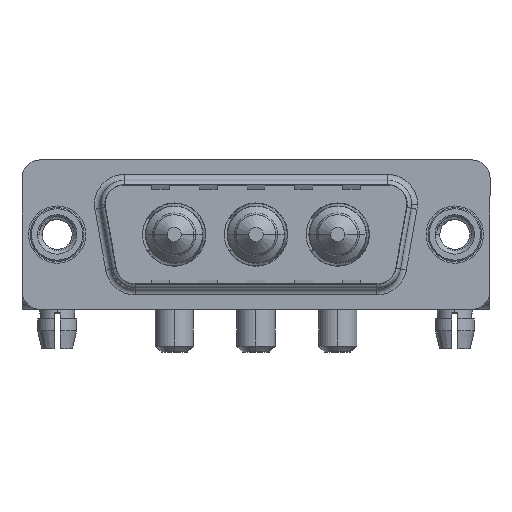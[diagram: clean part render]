
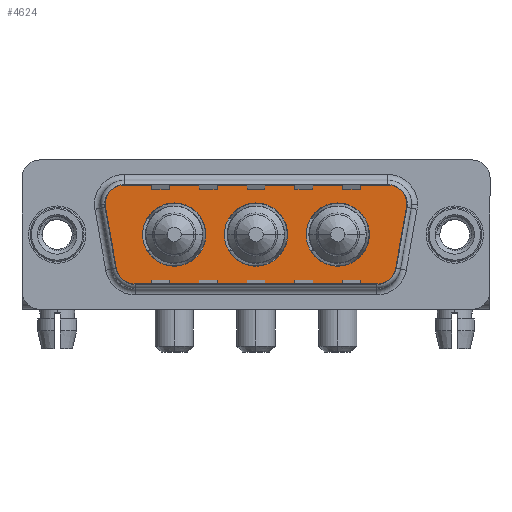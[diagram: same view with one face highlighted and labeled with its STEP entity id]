
A CAD part, top view. The second image highlights one B-rep face of the part: STEP entity #4624.
In plain terms, the highlighted planar face has unit normal (0, 0, 1).
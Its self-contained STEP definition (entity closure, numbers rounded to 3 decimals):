
#15 = EDGE_CURVE ( 'NONE', #15211, #13319, #9795, .T. ) ;
#98 = CARTESIAN_POINT ( 'NONE',  ( 5.411, 4.9, 0. ) ) ;
#566 = CIRCLE ( 'NONE', #9635, 2.65 ) ;
#804 = CARTESIAN_POINT ( 'NONE',  ( 4.464, -3.247, 0. ) ) ;
#961 = ORIENTED_EDGE ( 'NONE', *, *, #15995, .T. ) ;
#1162 = EDGE_LOOP ( 'NONE', ( #7619, #8279 ) ) ;
#1176 = ORIENTED_EDGE ( 'NONE', *, *, #10831, .T. ) ;
#1302 = DIRECTION ( 'NONE',  ( 0., 0., 1. ) ) ;
#1475 = EDGE_LOOP ( 'NONE', ( #9793, #8203 ) ) ;
#1520 = DIRECTION ( 'NONE',  ( 0., 0., 1. ) ) ;
#1812 = DIRECTION ( 'NONE',  ( 0., 0., 1. ) ) ;
#1900 = DIRECTION ( 'NONE',  ( 1., 0., 0. ) ) ;
#2204 = EDGE_CURVE ( 'NONE', #5105, #12135, #5934, .T. ) ;
#2297 = EDGE_CURVE ( 'NONE', #10391, #4183, #5661, .T. ) ;
#2346 = PLANE ( 'NONE',  #7996 ) ;
#2433 = EDGE_CURVE ( 'NONE', #5829, #15723, #12809, .T. ) ;
#2524 = CARTESIAN_POINT ( 'NONE',  ( 20.85, 0., 0. ) ) ;
#2596 = DIRECTION ( 'NONE',  ( 1., 0., 0. ) ) ;
#2720 = ORIENTED_EDGE ( 'NONE', *, *, #14276, .F. ) ;
#3393 = CARTESIAN_POINT ( 'NONE',  ( 23.5, 0., 0. ) ) ;
#3541 = VECTOR ( 'NONE', #15033, 1000. ) ;
#3607 = EDGE_CURVE ( 'NONE', #12135, #5105, #566, .T. ) ;
#3688 = DIRECTION ( 'NONE',  ( -1., 0., 0. ) ) ;
#3968 = FACE_BOUND ( 'NONE', #1475, .T. ) ;
#4048 = DIRECTION ( 'NONE',  ( 1., 0., 0. ) ) ;
#4058 = AXIS2_PLACEMENT_3D ( 'NONE', #6851, #8571, #6929 ) ;
#4127 = DIRECTION ( 'NONE',  ( 1., 0., 0. ) ) ;
#4183 = VERTEX_POINT ( 'NONE', #2524 ) ;
#4293 = CARTESIAN_POINT ( 'NONE',  ( 9.8, 0., 0. ) ) ;
#4350 = CARTESIAN_POINT ( 'NONE',  ( 9.8, 0., 0. ) ) ;
#4551 = VECTOR ( 'NONE', #9994, 1000. ) ;
#4624 = ADVANCED_FACE ( 'NONE', ( #3968, #9059, #15495, #14115 ), #2346, .T. ) ;
#4654 = DIRECTION ( 'NONE',  ( 1., 0., 0. ) ) ;
#4661 = AXIS2_PLACEMENT_3D ( 'NONE', #10235, #7649, #3688 ) ;
#4957 = ORIENTED_EDGE ( 'NONE', *, *, #14246, .T. ) ;
#5105 = VERTEX_POINT ( 'NONE', #8069 ) ;
#5158 = CARTESIAN_POINT ( 'NONE',  ( 6.434, -4.9, 0. ) ) ;
#5204 = CARTESIAN_POINT ( 'NONE',  ( 16.65, 0., 0. ) ) ;
#5661 = CIRCLE ( 'NONE', #10350, 2.65 ) ;
#5746 = EDGE_LOOP ( 'NONE', ( #15866, #4957, #961, #13502, #1176, #6097, #14659, #13693, #10417 ) ) ;
#5797 = DIRECTION ( 'NONE',  ( 1., 0., 0. ) ) ;
#5829 = VERTEX_POINT ( 'NONE', #9871 ) ;
#5934 = CIRCLE ( 'NONE', #13908, 2.65 ) ;
#6097 = ORIENTED_EDGE ( 'NONE', *, *, #15095, .T. ) ;
#6328 = DIRECTION ( 'NONE',  ( 0., 0., 1. ) ) ;
#6340 = EDGE_CURVE ( 'NONE', #13319, #12102, #13187, .T. ) ;
#6545 = DIRECTION ( 'NONE',  ( -1., 0., 0. ) ) ;
#6757 = CIRCLE ( 'NONE', #16381, 2.65 ) ;
#6778 = CARTESIAN_POINT ( 'NONE',  ( 3.441, 2.553, 0. ) ) ;
#6830 = CARTESIAN_POINT ( 'NONE',  ( 29.859, 2.553, 0. ) ) ;
#6851 = CARTESIAN_POINT ( 'NONE',  ( 5.411, 2.9, 0. ) ) ;
#6929 = DIRECTION ( 'NONE',  ( 1., 0., 0. ) ) ;
#7016 = CARTESIAN_POINT ( 'NONE',  ( 3.441, 2.553, 0. ) ) ;
#7040 = VERTEX_POINT ( 'NONE', #9364 ) ;
#7462 = LINE ( 'NONE', #15460, #13385 ) ;
#7537 = VERTEX_POINT ( 'NONE', #7994 ) ;
#7619 = ORIENTED_EDGE ( 'NONE', *, *, #2204, .F. ) ;
#7649 = DIRECTION ( 'NONE',  ( 0., 0., 1. ) ) ;
#7915 = LINE ( 'NONE', #98, #13825 ) ;
#7994 = CARTESIAN_POINT ( 'NONE',  ( 27.889, 4.9, 0. ) ) ;
#7995 = CARTESIAN_POINT ( 'NONE',  ( 16.65, 0., 0. ) ) ;
#7996 = AXIS2_PLACEMENT_3D ( 'NONE', #14363, #12837, #2596 ) ;
#8069 = CARTESIAN_POINT ( 'NONE',  ( 12.45, 0., 0. ) ) ;
#8203 = ORIENTED_EDGE ( 'NONE', *, *, #2433, .F. ) ;
#8231 = CARTESIAN_POINT ( 'NONE',  ( 29.889, 2.9, 0. ) ) ;
#8279 = ORIENTED_EDGE ( 'NONE', *, *, #3607, .F. ) ;
#8282 = VERTEX_POINT ( 'NONE', #13722 ) ;
#8382 = ORIENTED_EDGE ( 'NONE', *, *, #2297, .F. ) ;
#8571 = DIRECTION ( 'NONE',  ( 0., 0., 1. ) ) ;
#9059 = FACE_BOUND ( 'NONE', #16501, .T. ) ;
#9312 = DIRECTION ( 'NONE',  ( 0., 0., 1. ) ) ;
#9364 = CARTESIAN_POINT ( 'NONE',  ( 28.836, -3.247, 0. ) ) ;
#9485 = CARTESIAN_POINT ( 'NONE',  ( 19.3, 0., 0. ) ) ;
#9552 = CIRCLE ( 'NONE', #13934, 2. ) ;
#9635 = AXIS2_PLACEMENT_3D ( 'NONE', #4293, #1812, #1900 ) ;
#9786 = DIRECTION ( 'NONE',  ( 0., 0., 1. ) ) ;
#9793 = ORIENTED_EDGE ( 'NONE', *, *, #14463, .F. ) ;
#9795 = LINE ( 'NONE', #6778, #3541 ) ;
#9835 = LINE ( 'NONE', #6830, #4551 ) ;
#9871 = CARTESIAN_POINT ( 'NONE',  ( 14., 0., 0. ) ) ;
#9953 = CARTESIAN_POINT ( 'NONE',  ( 27.889, 2.9, 0. ) ) ;
#9994 = DIRECTION ( 'NONE',  ( 0.174, 0.985, 0. ) ) ;
#10235 = CARTESIAN_POINT ( 'NONE',  ( 6.434, -2.9, 0. ) ) ;
#10350 = AXIS2_PLACEMENT_3D ( 'NONE', #3393, #9786, #5797 ) ;
#10391 = VERTEX_POINT ( 'NONE', #15939 ) ;
#10417 = ORIENTED_EDGE ( 'NONE', *, *, #14865, .T. ) ;
#10548 = CARTESIAN_POINT ( 'NONE',  ( 26.866, -4.9, 0. ) ) ;
#10831 = EDGE_CURVE ( 'NONE', #7537, #8282, #7915, .T. ) ;
#11254 = DIRECTION ( 'NONE',  ( 0., 0., 1. ) ) ;
#11458 = AXIS2_PLACEMENT_3D ( 'NONE', #5204, #15782, #12778 ) ;
#11698 = CARTESIAN_POINT ( 'NONE',  ( 7.15, 0., 0. ) ) ;
#11872 = DIRECTION ( 'NONE',  ( 1., 0., 0. ) ) ;
#12102 = VERTEX_POINT ( 'NONE', #5158 ) ;
#12135 = VERTEX_POINT ( 'NONE', #11698 ) ;
#12165 = EDGE_CURVE ( 'NONE', #14042, #7040, #16889, .T. ) ;
#12690 = DIRECTION ( 'NONE',  ( -1., 0., 0. ) ) ;
#12715 = DIRECTION ( 'NONE',  ( 1., 0., 0. ) ) ;
#12778 = DIRECTION ( 'NONE',  ( 1., 0., 0. ) ) ;
#12809 = CIRCLE ( 'NONE', #11458, 2.65 ) ;
#12837 = DIRECTION ( 'NONE',  ( 0., 0., 1. ) ) ;
#13038 = DIRECTION ( 'NONE',  ( -1., 0., 0. ) ) ;
#13187 = CIRCLE ( 'NONE', #4661, 2. ) ;
#13299 = CARTESIAN_POINT ( 'NONE',  ( 29.859, 2.553, 0. ) ) ;
#13319 = VERTEX_POINT ( 'NONE', #804 ) ;
#13322 = CARTESIAN_POINT ( 'NONE',  ( 26.866, -2.9, 0. ) ) ;
#13385 = VECTOR ( 'NONE', #12715, 1000. ) ;
#13408 = AXIS2_PLACEMENT_3D ( 'NONE', #14314, #6328, #13038 ) ;
#13502 = ORIENTED_EDGE ( 'NONE', *, *, #15233, .T. ) ;
#13693 = ORIENTED_EDGE ( 'NONE', *, *, #6340, .T. ) ;
#13722 = CARTESIAN_POINT ( 'NONE',  ( 5.411, 4.9, 0. ) ) ;
#13825 = VECTOR ( 'NONE', #6545, 1000. ) ;
#13908 = AXIS2_PLACEMENT_3D ( 'NONE', #4350, #16227, #4048 ) ;
#13919 = CIRCLE ( 'NONE', #16125, 2.65 ) ;
#13934 = AXIS2_PLACEMENT_3D ( 'NONE', #9953, #11254, #12690 ) ;
#14042 = VERTEX_POINT ( 'NONE', #10548 ) ;
#14115 = FACE_OUTER_BOUND ( 'NONE', #5746, .T. ) ;
#14246 = EDGE_CURVE ( 'NONE', #7040, #16118, #9835, .T. ) ;
#14276 = EDGE_CURVE ( 'NONE', #4183, #10391, #6757, .T. ) ;
#14314 = CARTESIAN_POINT ( 'NONE',  ( 27.889, 2.9, 0. ) ) ;
#14363 = CARTESIAN_POINT ( 'NONE',  ( 26.866, -2.9, 0. ) ) ;
#14463 = EDGE_CURVE ( 'NONE', #15723, #5829, #13919, .T. ) ;
#14659 = ORIENTED_EDGE ( 'NONE', *, *, #15, .T. ) ;
#14865 = EDGE_CURVE ( 'NONE', #12102, #14042, #7462, .T. ) ;
#15033 = DIRECTION ( 'NONE',  ( 0.174, -0.985, 0. ) ) ;
#15091 = VERTEX_POINT ( 'NONE', #8231 ) ;
#15095 = EDGE_CURVE ( 'NONE', #8282, #15211, #15579, .T. ) ;
#15211 = VERTEX_POINT ( 'NONE', #7016 ) ;
#15233 = EDGE_CURVE ( 'NONE', #15091, #7537, #9552, .T. ) ;
#15460 = CARTESIAN_POINT ( 'NONE',  ( 6.434, -4.9, 0. ) ) ;
#15495 = FACE_BOUND ( 'NONE', #1162, .T. ) ;
#15579 = CIRCLE ( 'NONE', #4058, 2. ) ;
#15723 = VERTEX_POINT ( 'NONE', #9485 ) ;
#15773 = AXIS2_PLACEMENT_3D ( 'NONE', #13322, #1302, #11872 ) ;
#15782 = DIRECTION ( 'NONE',  ( 0., 0., 1. ) ) ;
#15866 = ORIENTED_EDGE ( 'NONE', *, *, #12165, .T. ) ;
#15939 = CARTESIAN_POINT ( 'NONE',  ( 26.15, 0., 0. ) ) ;
#15995 = EDGE_CURVE ( 'NONE', #16118, #15091, #16435, .T. ) ;
#16118 = VERTEX_POINT ( 'NONE', #13299 ) ;
#16125 = AXIS2_PLACEMENT_3D ( 'NONE', #7995, #9312, #4127 ) ;
#16227 = DIRECTION ( 'NONE',  ( 0., 0., 1. ) ) ;
#16381 = AXIS2_PLACEMENT_3D ( 'NONE', #16452, #1520, #4654 ) ;
#16435 = CIRCLE ( 'NONE', #13408, 2. ) ;
#16452 = CARTESIAN_POINT ( 'NONE',  ( 23.5, 0., 0. ) ) ;
#16501 = EDGE_LOOP ( 'NONE', ( #8382, #2720 ) ) ;
#16889 = CIRCLE ( 'NONE', #15773, 2. ) ;
